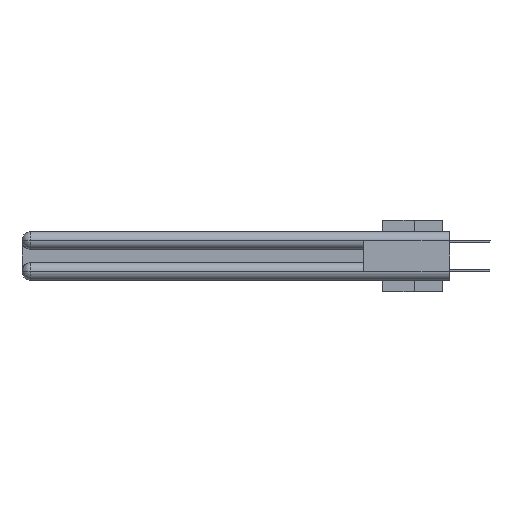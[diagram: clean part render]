
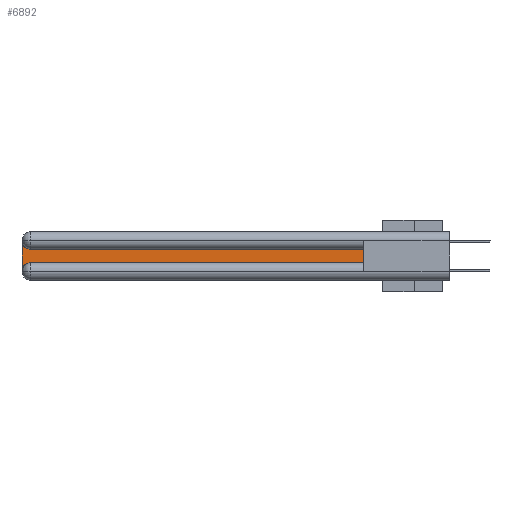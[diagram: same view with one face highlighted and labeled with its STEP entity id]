
A CAD part, left-side view. The second image highlights one B-rep face of the part: STEP entity #6892.
In plain terms, the highlighted planar face has unit normal (-1, 0, 0).
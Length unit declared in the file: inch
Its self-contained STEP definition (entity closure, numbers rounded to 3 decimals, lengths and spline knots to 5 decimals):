
#14 = CARTESIAN_POINT ( 'NONE',  ( 0.075, 3., -0.2175 ) ) ;
#189 = DIRECTION ( 'NONE',  ( 0., 0., -1. ) ) ;
#430 = VECTOR ( 'NONE', #17775, 39.37008 ) ;
#2114 = CARTESIAN_POINT ( 'NONE',  ( 0.075, 0.6, -0.2175 ) ) ;
#3226 = PLANE ( 'NONE',  #28174 ) ;
#3693 = EDGE_CURVE ( 'NONE', #29699, #28350, #30319, .T. ) ;
#3911 = LINE ( 'NONE', #8162, #430 ) ;
#4058 = LINE ( 'NONE', #14, #33784 ) ;
#4141 = AXIS2_PLACEMENT_3D ( 'NONE', #12623, #29022, #32168 ) ;
#5553 = CARTESIAN_POINT ( 'NONE',  ( 0.075, 3., -0.1225 ) ) ;
#6892 = ADVANCED_FACE ( 'NONE', ( #30961 ), #3226, .F. ) ;
#7014 = VERTEX_POINT ( 'NONE', #26152 ) ;
#7606 = ORIENTED_EDGE ( 'NONE', *, *, #19267, .T. ) ;
#8150 = EDGE_CURVE ( 'NONE', #15820, #7014, #9023, .T. ) ;
#8162 = CARTESIAN_POINT ( 'NONE',  ( 0.075, 0.6, -0.2175 ) ) ;
#8401 = ORIENTED_EDGE ( 'NONE', *, *, #35455, .T. ) ;
#8465 = VERTEX_POINT ( 'NONE', #33406 ) ;
#8487 = DIRECTION ( 'NONE',  ( 1., 0., 0. ) ) ;
#9023 = CIRCLE ( 'NONE', #4141, 0.06 ) ;
#9805 = AXIS2_PLACEMENT_3D ( 'NONE', #27527, #10683, #36086 ) ;
#10683 = DIRECTION ( 'NONE',  ( 1., 0., 0. ) ) ;
#12623 = CARTESIAN_POINT ( 'NONE',  ( 0.075, 2.94, -0.0625 ) ) ;
#14832 = DIRECTION ( 'NONE',  ( 0., 1., 0. ) ) ;
#15820 = VERTEX_POINT ( 'NONE', #17929 ) ;
#16293 = DIRECTION ( 'NONE',  ( 0., -1., 0. ) ) ;
#17775 = DIRECTION ( 'NONE',  ( 0., 0., 1. ) ) ;
#17799 = CARTESIAN_POINT ( 'NONE',  ( 0.075, 0.6, -0.1225 ) ) ;
#17814 = EDGE_CURVE ( 'NONE', #8465, #29699, #32530, .T. ) ;
#17929 = CARTESIAN_POINT ( 'NONE',  ( 0.075, 2.94, -0.1225 ) ) ;
#18131 = CARTESIAN_POINT ( 'NONE',  ( 0.075, 0.6, -0.1225 ) ) ;
#19267 = EDGE_CURVE ( 'NONE', #7014, #8465, #4058, .T. ) ;
#19489 = EDGE_CURVE ( 'NONE', #20140, #15820, #35546, .T. ) ;
#20140 = VERTEX_POINT ( 'NONE', #18131 ) ;
#21956 = ORIENTED_EDGE ( 'NONE', *, *, #3693, .T. ) ;
#22086 = DIRECTION ( 'NONE',  ( 0., 0., -1. ) ) ;
#22933 = VECTOR ( 'NONE', #16293, 39.37008 ) ;
#25169 = EDGE_LOOP ( 'NONE', ( #28720, #27759, #7606, #33694, #21956, #8401 ) ) ;
#26152 = CARTESIAN_POINT ( 'NONE',  ( 0.075, 3., -0.0625 ) ) ;
#27527 = CARTESIAN_POINT ( 'NONE',  ( 0.075, 2.94, -0.2775 ) ) ;
#27759 = ORIENTED_EDGE ( 'NONE', *, *, #8150, .T. ) ;
#28101 = VECTOR ( 'NONE', #14832, 39.37008 ) ;
#28174 = AXIS2_PLACEMENT_3D ( 'NONE', #5553, #8487, #189 ) ;
#28350 = VERTEX_POINT ( 'NONE', #2114 ) ;
#28720 = ORIENTED_EDGE ( 'NONE', *, *, #19489, .T. ) ;
#29022 = DIRECTION ( 'NONE',  ( 1., 0., 0. ) ) ;
#29699 = VERTEX_POINT ( 'NONE', #35321 ) ;
#30319 = LINE ( 'NONE', #32998, #22933 ) ;
#30961 = FACE_OUTER_BOUND ( 'NONE', #25169, .T. ) ;
#32168 = DIRECTION ( 'NONE',  ( 0., 0., -1. ) ) ;
#32530 = CIRCLE ( 'NONE', #9805, 0.06 ) ;
#32998 = CARTESIAN_POINT ( 'NONE',  ( 0.075, 0.6, -0.2175 ) ) ;
#33406 = CARTESIAN_POINT ( 'NONE',  ( 0.075, 3., -0.2775 ) ) ;
#33694 = ORIENTED_EDGE ( 'NONE', *, *, #17814, .T. ) ;
#33784 = VECTOR ( 'NONE', #22086, 39.37008 ) ;
#35321 = CARTESIAN_POINT ( 'NONE',  ( 0.075, 2.94, -0.2175 ) ) ;
#35455 = EDGE_CURVE ( 'NONE', #28350, #20140, #3911, .T. ) ;
#35546 = LINE ( 'NONE', #17799, #28101 ) ;
#36086 = DIRECTION ( 'NONE',  ( 0., 0., -1. ) ) ;
